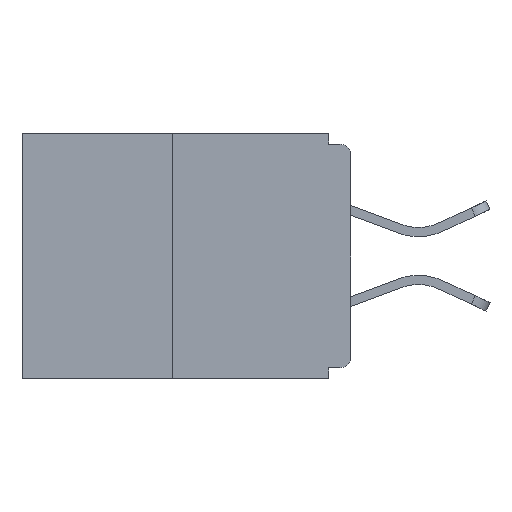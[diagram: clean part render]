
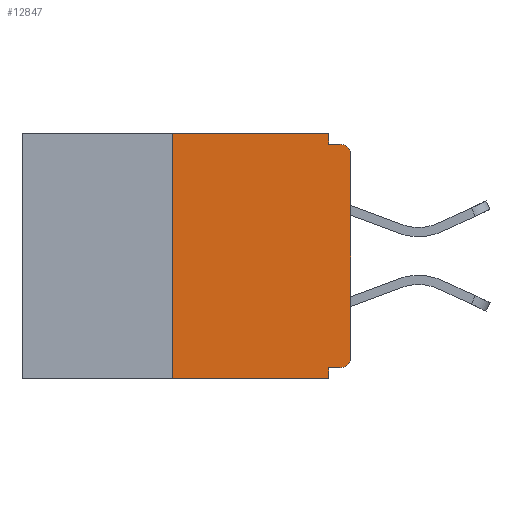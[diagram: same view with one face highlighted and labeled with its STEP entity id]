
A CAD part, left-side view. The second image highlights one B-rep face of the part: STEP entity #12847.
In plain terms, the highlighted planar face has unit normal (-1, 0, 0).
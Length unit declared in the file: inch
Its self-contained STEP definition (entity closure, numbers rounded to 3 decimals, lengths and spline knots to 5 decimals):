
#165 = CARTESIAN_POINT ( 'NONE',  ( 0., 0.015, -0.313 ) ) ;
#238 = ORIENTED_EDGE ( 'NONE', *, *, #2425, .T. ) ;
#255 = LINE ( 'NONE', #8174, #13453 ) ;
#274 = EDGE_CURVE ( 'NONE', #16593, #12413, #13627, .T. ) ;
#502 = DIRECTION ( 'NONE',  ( -1., 0., 0. ) ) ;
#541 = AXIS2_PLACEMENT_3D ( 'NONE', #9832, #3296, #1804 ) ;
#551 = VECTOR ( 'NONE', #16446, 39.37008 ) ;
#1461 = AXIS2_PLACEMENT_3D ( 'NONE', #165, #6751, #4105 ) ;
#1766 = CARTESIAN_POINT ( 'NONE',  ( 0., 0.031, -0.343 ) ) ;
#1804 = DIRECTION ( 'NONE',  ( 0., 0., -1. ) ) ;
#1868 = CARTESIAN_POINT ( 'NONE',  ( 0., 0.031, -0.015 ) ) ;
#1985 = DIRECTION ( 'NONE',  ( 0., 0., -1. ) ) ;
#2363 = ORIENTED_EDGE ( 'NONE', *, *, #6692, .T. ) ;
#2425 = EDGE_CURVE ( 'NONE', #8591, #16407, #2754, .T. ) ;
#2439 = VERTEX_POINT ( 'NONE', #1868 ) ;
#2461 = ORIENTED_EDGE ( 'NONE', *, *, #2594, .F. ) ;
#2573 = VECTOR ( 'NONE', #3594, 39.37008 ) ;
#2594 = EDGE_CURVE ( 'NONE', #11156, #2439, #3967, .T. ) ;
#2754 = CIRCLE ( 'NONE', #6444, 0.015 ) ;
#3029 = LINE ( 'NONE', #12040, #16520 ) ;
#3115 = VERTEX_POINT ( 'NONE', #14270 ) ;
#3133 = DIRECTION ( 'NONE',  ( 0., 0., -1. ) ) ;
#3296 = DIRECTION ( 'NONE',  ( 1., 0., 0. ) ) ;
#3594 = DIRECTION ( 'NONE',  ( 0., -1., 0. ) ) ;
#3794 = VECTOR ( 'NONE', #16648, 39.37008 ) ;
#3967 = LINE ( 'NONE', #13786, #551 ) ;
#4105 = DIRECTION ( 'NONE',  ( 0., 0., -1. ) ) ;
#4197 = CARTESIAN_POINT ( 'NONE',  ( 0., 0., 0. ) ) ;
#4226 = DIRECTION ( 'NONE',  ( 0., 1., 0. ) ) ;
#4586 = ORIENTED_EDGE ( 'NONE', *, *, #9679, .F. ) ;
#4689 = CARTESIAN_POINT ( 'NONE',  ( 0., 0.031, -0.343 ) ) ;
#4957 = VERTEX_POINT ( 'NONE', #6836 ) ;
#5119 = DIRECTION ( 'NONE',  ( 0., -1., 0. ) ) ;
#5125 = ORIENTED_EDGE ( 'NONE', *, *, #5302, .F. ) ;
#5302 = EDGE_CURVE ( 'NONE', #2439, #16407, #255, .T. ) ;
#5440 = ORIENTED_EDGE ( 'NONE', *, *, #274, .T. ) ;
#5459 = ORIENTED_EDGE ( 'NONE', *, *, #8251, .F. ) ;
#5681 = DIRECTION ( 'NONE',  ( 0., 0., 1. ) ) ;
#5969 = EDGE_LOOP ( 'NONE', ( #13209, #5459, #5440, #4586, #14195, #9985, #2363, #238, #5125, #2461 ) ) ;
#6297 = LINE ( 'NONE', #4197, #13205 ) ;
#6360 = CIRCLE ( 'NONE', #1461, 0.015 ) ;
#6444 = AXIS2_PLACEMENT_3D ( 'NONE', #13450, #502, #3133 ) ;
#6564 = CARTESIAN_POINT ( 'NONE',  ( 0., 0.031, -0.328 ) ) ;
#6692 = EDGE_CURVE ( 'NONE', #4957, #8591, #6297, .T. ) ;
#6751 = DIRECTION ( 'NONE',  ( -1., 0., 0. ) ) ;
#6776 = CARTESIAN_POINT ( 'NONE',  ( 0., 0.015, -0.015 ) ) ;
#6836 = CARTESIAN_POINT ( 'NONE',  ( 0., 0., -0.313 ) ) ;
#7488 = CARTESIAN_POINT ( 'NONE',  ( 0., 0.46, 0. ) ) ;
#7616 = FACE_OUTER_BOUND ( 'NONE', #5969, .T. ) ;
#7691 = CARTESIAN_POINT ( 'NONE',  ( 0., 0.25, 0. ) ) ;
#7700 = VERTEX_POINT ( 'NONE', #6564 ) ;
#7890 = LINE ( 'NONE', #7691, #3794 ) ;
#8174 = CARTESIAN_POINT ( 'NONE',  ( 0., 0., -0.015 ) ) ;
#8251 = EDGE_CURVE ( 'NONE', #16593, #3115, #7890, .T. ) ;
#8508 = PLANE ( 'NONE',  #541 ) ;
#8591 = VERTEX_POINT ( 'NONE', #13750 ) ;
#9679 = EDGE_CURVE ( 'NONE', #7700, #12413, #11316, .T. ) ;
#9832 = CARTESIAN_POINT ( 'NONE',  ( 0., 0.46, 0. ) ) ;
#9985 = ORIENTED_EDGE ( 'NONE', *, *, #14248, .T. ) ;
#10397 = CARTESIAN_POINT ( 'NONE',  ( 0., 0.46, -0.343 ) ) ;
#10642 = CARTESIAN_POINT ( 'NONE',  ( 0., 0.25, -0.343 ) ) ;
#10858 = DIRECTION ( 'NONE',  ( 0., -1., 0. ) ) ;
#11156 = VERTEX_POINT ( 'NONE', #15884 ) ;
#11311 = EDGE_CURVE ( 'NONE', #3115, #11156, #13971, .T. ) ;
#11316 = LINE ( 'NONE', #1766, #16422 ) ;
#11559 = CARTESIAN_POINT ( 'NONE',  ( 0., 0.015, -0.328 ) ) ;
#12040 = CARTESIAN_POINT ( 'NONE',  ( 0., 0., -0.328 ) ) ;
#12413 = VERTEX_POINT ( 'NONE', #4689 ) ;
#12643 = VERTEX_POINT ( 'NONE', #11559 ) ;
#12847 = ADVANCED_FACE ( 'NONE', ( #7616 ), #8508, .F. ) ;
#13205 = VECTOR ( 'NONE', #5681, 39.37008 ) ;
#13209 = ORIENTED_EDGE ( 'NONE', *, *, #11311, .F. ) ;
#13450 = CARTESIAN_POINT ( 'NONE',  ( 0., 0.015, -0.03 ) ) ;
#13453 = VECTOR ( 'NONE', #10858, 39.37008 ) ;
#13627 = LINE ( 'NONE', #10397, #15868 ) ;
#13750 = CARTESIAN_POINT ( 'NONE',  ( 0., 0., -0.03 ) ) ;
#13786 = CARTESIAN_POINT ( 'NONE',  ( 0., 0.031, 0. ) ) ;
#13971 = LINE ( 'NONE', #7488, #2573 ) ;
#14195 = ORIENTED_EDGE ( 'NONE', *, *, #15863, .F. ) ;
#14248 = EDGE_CURVE ( 'NONE', #12643, #4957, #6360, .T. ) ;
#14270 = CARTESIAN_POINT ( 'NONE',  ( 0., 0.25, 0. ) ) ;
#15863 = EDGE_CURVE ( 'NONE', #12643, #7700, #3029, .T. ) ;
#15868 = VECTOR ( 'NONE', #5119, 39.37008 ) ;
#15884 = CARTESIAN_POINT ( 'NONE',  ( 0., 0.031, 0. ) ) ;
#16407 = VERTEX_POINT ( 'NONE', #6776 ) ;
#16422 = VECTOR ( 'NONE', #1985, 39.37008 ) ;
#16446 = DIRECTION ( 'NONE',  ( 0., 0., -1. ) ) ;
#16520 = VECTOR ( 'NONE', #4226, 39.37008 ) ;
#16593 = VERTEX_POINT ( 'NONE', #10642 ) ;
#16648 = DIRECTION ( 'NONE',  ( 0., 0., 1. ) ) ;
